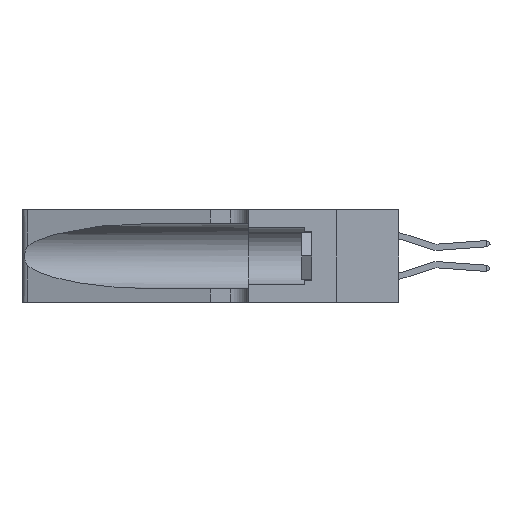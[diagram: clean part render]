
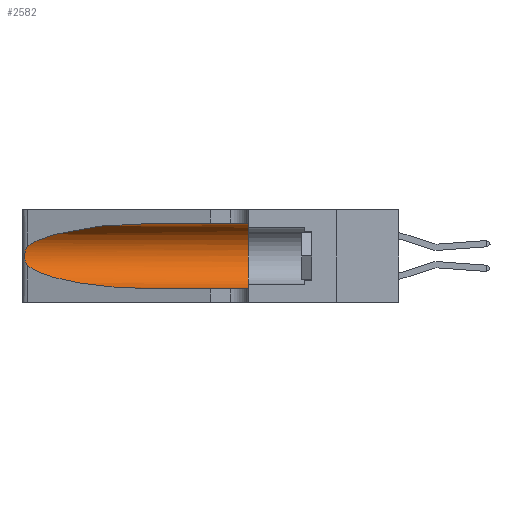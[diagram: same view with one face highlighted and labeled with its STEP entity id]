
A CAD part, left-side view. The second image highlights one B-rep face of the part: STEP entity #2582.
In plain terms, the highlighted cylindrical face has radius 3.308 mm (diameter 6.617 mm), a partial arc.
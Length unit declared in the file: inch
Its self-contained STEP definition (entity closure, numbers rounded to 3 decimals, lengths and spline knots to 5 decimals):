
#1199 = VERTEX_POINT ( 'NONE', #19795 ) ;
#2144 = CARTESIAN_POINT ( 'NONE',  ( 0.25555, 1.22993, 0.14849 ) ) ;
#2582 = ADVANCED_FACE ( 'NONE', ( #22695 ), #15857, .F. ) ;
#2686 = CARTESIAN_POINT ( 'NONE',  ( 0.2373, 1.15595, 0.28018 ) ) ;
#5342 = CARTESIAN_POINT ( 'NONE',  ( 0.1305, 0.72297, 0.31525 ) ) ;
#5763 = CARTESIAN_POINT ( 'NONE',  ( 0.26017, 1.23833, 0.17102 ) ) ;
#5779 = EDGE_CURVE ( 'NONE', #1199, #36118, #37053, .T. ) ;
#6659 = DIRECTION ( 'NONE',  ( 0., 1., 0. ) ) ;
#7535 = CARTESIAN_POINT ( 'NONE',  ( 0.25487, 1.22718, 0.22369 ) ) ;
#7557 = EDGE_CURVE ( 'NONE', #30151, #24045, #32304, .T. ) ;
#8130 = CARTESIAN_POINT ( 'NONE',  ( 0.26075, 1.23896, 0.178 ) ) ;
#9195 = ORIENTED_EDGE ( 'NONE', *, *, #7557, .T. ) ;
#9529 = EDGE_CURVE ( 'NONE', #26833, #30151, #40889, .T. ) ;
#10599 = CARTESIAN_POINT ( 'NONE',  ( 0.1305, 0.35, 0.185 ) ) ;
#11442 = CARTESIAN_POINT ( 'NONE',  ( 0.1305, 0.72297, 0.05475 ) ) ;
#11532 = CIRCLE ( 'NONE', #13573, 0.13025 ) ;
#12654 = LINE ( 'NONE', #24863, #42217 ) ;
#12842 = CARTESIAN_POINT ( 'NONE',  ( 0.1305, 0.35, 0.31525 ) ) ;
#13573 = AXIS2_PLACEMENT_3D ( 'NONE', #10599, #6659, #17384 ) ;
#14364 = CARTESIAN_POINT ( 'NONE',  ( 0.25555, 1.22994, 0.2215 ) ) ;
#14802 = CARTESIAN_POINT ( 'NONE',  ( 0.2373, 1.15595, 0.08982 ) ) ;
#15186 = ORIENTED_EDGE ( 'NONE', *, *, #9529, .T. ) ;
#15251 = CARTESIAN_POINT ( 'NONE',  ( 0.25854, 1.2359, 0.20912 ) ) ;
#15857 = CYLINDRICAL_SURFACE ( 'NONE', #41338, 0.13025 ) ;
#17384 = DIRECTION ( 'NONE',  ( 0., 0., 1. ) ) ;
#17538 = DIRECTION ( 'NONE',  ( 0., -1., 0. ) ) ;
#18169 = CARTESIAN_POINT ( 'NONE',  ( 0.26018, 1.23835, 0.19895 ) ) ;
#18306 = CARTESIAN_POINT ( 'NONE',  ( 0.1305, 0.72297, 0.05475 ) ) ;
#18428 = EDGE_CURVE ( 'NONE', #36118, #26833, #33055, .T. ) ;
#18503 = DIRECTION ( 'NONE',  ( 0., -1., 0. ) ) ;
#18920 = CARTESIAN_POINT ( 'NONE',  ( 0.25789, 1.23486, 0.15765 ) ) ;
#19795 = CARTESIAN_POINT ( 'NONE',  ( 0.1305, 0.72297, 0.31525 ) ) ;
#22306 = CARTESIAN_POINT ( 'NONE',  ( 0.25639, 1.23186, 0.15144 ) ) ;
#22695 = FACE_OUTER_BOUND ( 'NONE', #42515, .T. ) ;
#24045 = VERTEX_POINT ( 'NONE', #25430 ) ;
#24160 = CARTESIAN_POINT ( 'NONE',  ( 0.1305, 1.61858, 0.185 ) ) ;
#24863 = CARTESIAN_POINT ( 'NONE',  ( 0.1305, 1.61858, 0.31525 ) ) ;
#25430 = CARTESIAN_POINT ( 'NONE',  ( 0.1305, 0.35, 0.05475 ) ) ;
#26227 = EDGE_CURVE ( 'NONE', #43289, #24045, #11532, .T. ) ;
#26833 = VERTEX_POINT ( 'NONE', #35988 ) ;
#27544 = DIRECTION ( 'NONE',  ( 0., 0., -1. ) ) ;
#28033 = CARTESIAN_POINT ( 'NONE',  ( 0.18966, 0.96281, 0.05475 ) ) ;
#28270 = DIRECTION ( 'NONE',  ( 0., -1., 0. ) ) ;
#28664 = CARTESIAN_POINT ( 'NONE',  ( 0.1305, 1.61858, 0.05475 ) ) ;
#28884 = ORIENTED_EDGE ( 'NONE', *, *, #18428, .T. ) ;
#29023 = CARTESIAN_POINT ( 'NONE',  ( 0.25487, 1.22718, 0.22369 ) ) ;
#29436 = EDGE_CURVE ( 'NONE', #1199, #43289, #12654, .T. ) ;
#30151 = VERTEX_POINT ( 'NONE', #11442 ) ;
#30621 = CARTESIAN_POINT ( 'NONE',  ( 0.25487, 1.22718, 0.22369 ) ) ;
#31587 = CARTESIAN_POINT ( 'NONE',  ( 0.26075, 1.23896, 0.19203 ) ) ;
#31785 = VECTOR ( 'NONE', #18503, 39.37008 ) ;
#32304 = LINE ( 'NONE', #28664, #31785 ) ;
#32318 = CARTESIAN_POINT ( 'NONE',  ( 0.25856, 1.23593, 0.16098 ) ) ;
#33055 = B_SPLINE_CURVE_WITH_KNOTS ( 'NONE', 3,
 ( #7535, #14364, #41336, #34802, #15251, #18169, #31587, #8130, #5763, #32318, #18920, #22306, #2144, #35846 ),
 .UNSPECIFIED., .F., .F.,
 ( 4, 2, 2, 2, 2, 2, 4 ),
 ( 0., 0.00027, 0.00053, 0.00107, 0.0016, 0.00187, 0.00214 ),
 .UNSPECIFIED. ) ;
#33313 = CARTESIAN_POINT ( 'NONE',  ( 0.18966, 0.96281, 0.31525 ) ) ;
#34802 = CARTESIAN_POINT ( 'NONE',  ( 0.25787, 1.23484, 0.2124 ) ) ;
#35157 = ORIENTED_EDGE ( 'NONE', *, *, #5779, .T. ) ;
#35846 = CARTESIAN_POINT ( 'NONE',  ( 0.25487, 1.22718, 0.14631 ) ) ;
#35988 = CARTESIAN_POINT ( 'NONE',  ( 0.25487, 1.22718, 0.14631 ) ) ;
#36118 = VERTEX_POINT ( 'NONE', #30621 ) ;
#37053 =( BOUNDED_CURVE ( )  B_SPLINE_CURVE ( 3, ( #5342, #33313, #2686, #29023 ),
 .UNSPECIFIED., .F., .T. ) 
 B_SPLINE_CURVE_WITH_KNOTS ( ( 4, 4 ),
 ( 1.5708, 2.84003 ),
 .UNSPECIFIED. ) 
 CURVE ( )  GEOMETRIC_REPRESENTATION_ITEM ( )  RATIONAL_B_SPLINE_CURVE ( ( 1., 0.87, 0.87, 1. ) ) 
 REPRESENTATION_ITEM ( '' )  );
#37509 = ORIENTED_EDGE ( 'NONE', *, *, #26227, .F. ) ;
#37728 = CARTESIAN_POINT ( 'NONE',  ( 0.25487, 1.22718, 0.14631 ) ) ;
#40889 =( BOUNDED_CURVE ( )  B_SPLINE_CURVE ( 3, ( #37728, #14802, #28033, #18306 ),
 .UNSPECIFIED., .F., .T. ) 
 B_SPLINE_CURVE_WITH_KNOTS ( ( 4, 4 ),
 ( 3.44316, 4.71239 ),
 .UNSPECIFIED. ) 
 CURVE ( )  GEOMETRIC_REPRESENTATION_ITEM ( )  RATIONAL_B_SPLINE_CURVE ( ( 1., 0.87, 0.87, 1. ) ) 
 REPRESENTATION_ITEM ( '' )  );
#41336 = CARTESIAN_POINT ( 'NONE',  ( 0.25639, 1.23184, 0.21858 ) ) ;
#41338 = AXIS2_PLACEMENT_3D ( 'NONE', #24160, #17538, #27544 ) ;
#42217 = VECTOR ( 'NONE', #28270, 39.37008 ) ;
#42515 = EDGE_LOOP ( 'NONE', ( #35157, #28884, #15186, #9195, #37509, #42616 ) ) ;
#42616 = ORIENTED_EDGE ( 'NONE', *, *, #29436, .F. ) ;
#43289 = VERTEX_POINT ( 'NONE', #12842 ) ;
